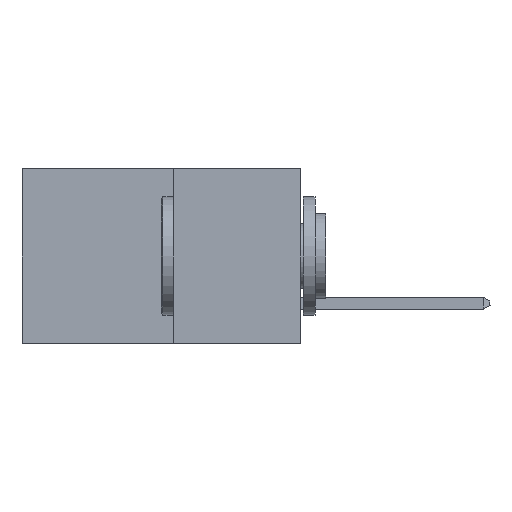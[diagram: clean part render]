
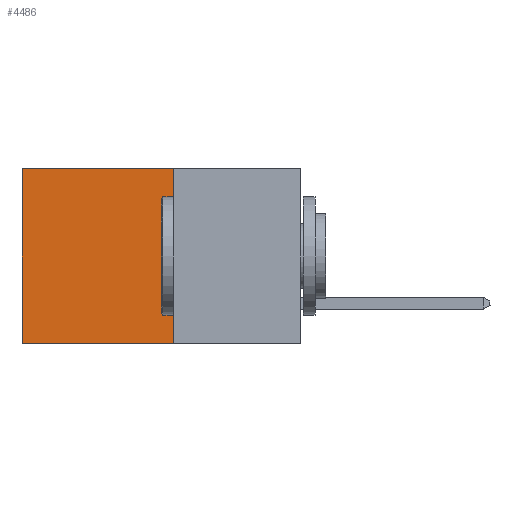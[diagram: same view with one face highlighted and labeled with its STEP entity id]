
A CAD part, left-side view. The second image highlights one B-rep face of the part: STEP entity #4486.
In plain terms, the highlighted planar face has unit normal (-1, 0, 0).
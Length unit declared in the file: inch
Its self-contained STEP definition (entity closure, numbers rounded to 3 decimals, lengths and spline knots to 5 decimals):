
#209 = VECTOR ( 'NONE', #26811, 39.37008 ) ;
#1014 = LINE ( 'NONE', #24139, #209 ) ;
#1492 = EDGE_CURVE ( 'NONE', #27676, #12873, #1014, .T. ) ;
#1587 = ORIENTED_EDGE ( 'NONE', *, *, #31837, .F. ) ;
#2720 = CARTESIAN_POINT ( 'NONE',  ( 0.277, 0.27, -0.37 ) ) ;
#4015 = LINE ( 'NONE', #30041, #23914 ) ;
#4486 = ADVANCED_FACE ( 'NONE', ( #21528 ), #17620, .F. ) ;
#4976 = CARTESIAN_POINT ( 'NONE',  ( 0.277, 0.59, -0.37 ) ) ;
#5057 = LINE ( 'NONE', #19669, #18045 ) ;
#5890 = EDGE_CURVE ( 'NONE', #12873, #18163, #4015, .T. ) ;
#11318 = CARTESIAN_POINT ( 'NONE',  ( 0.277, 0.59, 0. ) ) ;
#12331 = AXIS2_PLACEMENT_3D ( 'NONE', #17060, #16996, #16985 ) ;
#12873 = VERTEX_POINT ( 'NONE', #11318 ) ;
#13975 = EDGE_LOOP ( 'NONE', ( #19222, #1587, #15656, #33070 ) ) ;
#14584 = DIRECTION ( 'NONE',  ( 0., 0., -1. ) ) ;
#15656 = ORIENTED_EDGE ( 'NONE', *, *, #17260, .F. ) ;
#16985 = DIRECTION ( 'NONE',  ( 0., 0., -1. ) ) ;
#16996 = DIRECTION ( 'NONE',  ( 1., 0., 0. ) ) ;
#17060 = CARTESIAN_POINT ( 'NONE',  ( 0.277, 0.27, -0.37 ) ) ;
#17260 = EDGE_CURVE ( 'NONE', #27676, #19770, #5057, .T. ) ;
#17620 = PLANE ( 'NONE',  #12331 ) ;
#18045 = VECTOR ( 'NONE', #14584, 39.37008 ) ;
#18163 = VERTEX_POINT ( 'NONE', #4976 ) ;
#19222 = ORIENTED_EDGE ( 'NONE', *, *, #5890, .T. ) ;
#19669 = CARTESIAN_POINT ( 'NONE',  ( 0.277, 0.27, -0.37 ) ) ;
#19770 = VERTEX_POINT ( 'NONE', #2720 ) ;
#20150 = DIRECTION ( 'NONE',  ( 0., 1., 0. ) ) ;
#21122 = CARTESIAN_POINT ( 'NONE',  ( 0.277, 0.27, 0. ) ) ;
#21528 = FACE_OUTER_BOUND ( 'NONE', #13975, .T. ) ;
#23728 = VECTOR ( 'NONE', #20150, 39.37008 ) ;
#23914 = VECTOR ( 'NONE', #31420, 39.37008 ) ;
#24139 = CARTESIAN_POINT ( 'NONE',  ( 0.277, 0.27, 0. ) ) ;
#26811 = DIRECTION ( 'NONE',  ( 0., 1., 0. ) ) ;
#27676 = VERTEX_POINT ( 'NONE', #21122 ) ;
#30041 = CARTESIAN_POINT ( 'NONE',  ( 0.277, 0.59, -0.37 ) ) ;
#30380 = CARTESIAN_POINT ( 'NONE',  ( 0.277, 0.27, -0.37 ) ) ;
#30510 = LINE ( 'NONE', #30380, #23728 ) ;
#31420 = DIRECTION ( 'NONE',  ( 0., 0., -1. ) ) ;
#31837 = EDGE_CURVE ( 'NONE', #19770, #18163, #30510, .T. ) ;
#33070 = ORIENTED_EDGE ( 'NONE', *, *, #1492, .T. ) ;
